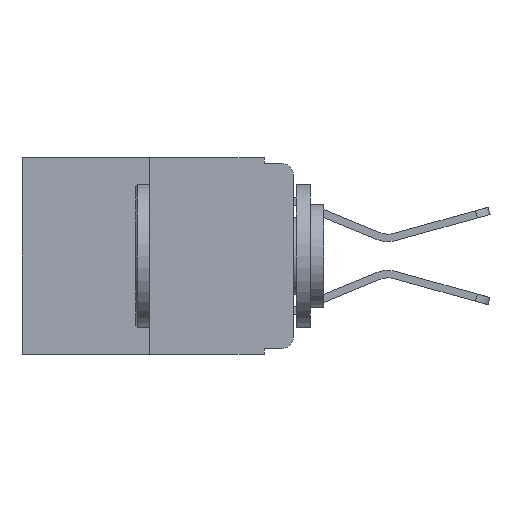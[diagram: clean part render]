
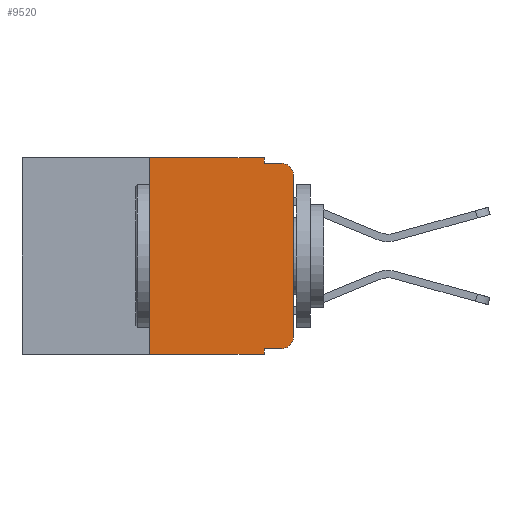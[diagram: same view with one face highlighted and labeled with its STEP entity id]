
A CAD part, left-side view. The second image highlights one B-rep face of the part: STEP entity #9520.
In plain terms, the highlighted planar face has unit normal (-1, 0, 0).
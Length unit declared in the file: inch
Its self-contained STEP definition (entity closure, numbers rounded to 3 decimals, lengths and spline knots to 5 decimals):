
#51 = DIRECTION ( 'NONE',  ( 0., 0., -1. ) ) ;
#485 = VECTOR ( 'NONE', #3410, 39.37008 ) ;
#599 = CARTESIAN_POINT ( 'NONE',  ( 0., 0.473, 0. ) ) ;
#651 = DIRECTION ( 'NONE',  ( 0., 0., 1. ) ) ;
#679 = VERTEX_POINT ( 'NONE', #16897 ) ;
#790 = EDGE_LOOP ( 'NONE', ( #5676, #9482, #6109, #9909, #6571, #10332, #13856, #10764, #17760, #11168 ) ) ;
#1125 = LINE ( 'NONE', #15892, #15273 ) ;
#1356 = CARTESIAN_POINT ( 'NONE',  ( 0., 0.051, -0.333 ) ) ;
#2352 = FACE_OUTER_BOUND ( 'NONE', #790, .T. ) ;
#2386 = VECTOR ( 'NONE', #51, 39.37008 ) ;
#2667 = CARTESIAN_POINT ( 'NONE',  ( 0., 0.25, 0. ) ) ;
#2975 = DIRECTION ( 'NONE',  ( 0., 0., -1. ) ) ;
#3064 = AXIS2_PLACEMENT_3D ( 'NONE', #599, #6646, #16149 ) ;
#3410 = DIRECTION ( 'NONE',  ( 0., -1., 0. ) ) ;
#3699 = CARTESIAN_POINT ( 'NONE',  ( 0., 0.25, -0.343 ) ) ;
#4577 = EDGE_CURVE ( 'NONE', #679, #4791, #16832, .T. ) ;
#4617 = CARTESIAN_POINT ( 'NONE',  ( 0., 0.051, -0.343 ) ) ;
#4672 = CARTESIAN_POINT ( 'NONE',  ( 0., 0., -0.03 ) ) ;
#4791 = VERTEX_POINT ( 'NONE', #8675 ) ;
#5560 = EDGE_CURVE ( 'NONE', #17378, #679, #10414, .T. ) ;
#5676 = ORIENTED_EDGE ( 'NONE', *, *, #11182, .T. ) ;
#6109 = ORIENTED_EDGE ( 'NONE', *, *, #9392, .F. ) ;
#6330 = VERTEX_POINT ( 'NONE', #2667 ) ;
#6506 = EDGE_CURVE ( 'NONE', #17378, #12170, #6618, .T. ) ;
#6571 = ORIENTED_EDGE ( 'NONE', *, *, #9517, .F. ) ;
#6618 = LINE ( 'NONE', #10194, #13485 ) ;
#6646 = DIRECTION ( 'NONE',  ( 1., 0., 0. ) ) ;
#6803 = CARTESIAN_POINT ( 'NONE',  ( 0., 0.02, -0.03 ) ) ;
#7354 = CARTESIAN_POINT ( 'NONE',  ( 0., 0., 0. ) ) ;
#7487 = EDGE_CURVE ( 'NONE', #8853, #6330, #9915, .T. ) ;
#7873 = CARTESIAN_POINT ( 'NONE',  ( 0., 0.473, -0.343 ) ) ;
#8002 = LINE ( 'NONE', #7873, #485 ) ;
#8190 = DIRECTION ( 'NONE',  ( -1., 0., 0. ) ) ;
#8303 = DIRECTION ( 'NONE',  ( 0., 0., -1. ) ) ;
#8476 = EDGE_CURVE ( 'NONE', #15116, #13767, #13199, .T. ) ;
#8675 = CARTESIAN_POINT ( 'NONE',  ( 0., 0., -0.313 ) ) ;
#8853 = VERTEX_POINT ( 'NONE', #3699 ) ;
#9007 = CARTESIAN_POINT ( 'NONE',  ( 0., 0.051, 0. ) ) ;
#9392 = EDGE_CURVE ( 'NONE', #13767, #12558, #1125, .T. ) ;
#9461 = CARTESIAN_POINT ( 'NONE',  ( 0., 0.473, 0. ) ) ;
#9482 = ORIENTED_EDGE ( 'NONE', *, *, #10296, .T. ) ;
#9517 = EDGE_CURVE ( 'NONE', #6330, #15116, #10914, .T. ) ;
#9520 = ADVANCED_FACE ( 'NONE', ( #2352 ), #14814, .F. ) ;
#9909 = ORIENTED_EDGE ( 'NONE', *, *, #8476, .F. ) ;
#9915 = LINE ( 'NONE', #16144, #15753 ) ;
#9991 = VECTOR ( 'NONE', #12642, 39.37008 ) ;
#10194 = CARTESIAN_POINT ( 'NONE',  ( 0., 0.051, 0. ) ) ;
#10296 = EDGE_CURVE ( 'NONE', #12800, #12558, #15470, .T. ) ;
#10332 = ORIENTED_EDGE ( 'NONE', *, *, #7487, .F. ) ;
#10414 = LINE ( 'NONE', #15318, #9991 ) ;
#10456 = VECTOR ( 'NONE', #11479, 39.37008 ) ;
#10764 = ORIENTED_EDGE ( 'NONE', *, *, #6506, .F. ) ;
#10914 = LINE ( 'NONE', #9461, #13587 ) ;
#11168 = ORIENTED_EDGE ( 'NONE', *, *, #4577, .T. ) ;
#11182 = EDGE_CURVE ( 'NONE', #4791, #12800, #14404, .T. ) ;
#11479 = DIRECTION ( 'NONE',  ( 0., 0., 1. ) ) ;
#11923 = AXIS2_PLACEMENT_3D ( 'NONE', #6803, #16303, #8303 ) ;
#12170 = VERTEX_POINT ( 'NONE', #4617 ) ;
#12172 = DIRECTION ( 'NONE',  ( 0., -1., 0. ) ) ;
#12365 = CARTESIAN_POINT ( 'NONE',  ( 0., 0.02, -0.01 ) ) ;
#12558 = VERTEX_POINT ( 'NONE', #12365 ) ;
#12642 = DIRECTION ( 'NONE',  ( 0., -1., 0. ) ) ;
#12800 = VERTEX_POINT ( 'NONE', #4672 ) ;
#13199 = LINE ( 'NONE', #9007, #2386 ) ;
#13485 = VECTOR ( 'NONE', #2975, 39.37008 ) ;
#13587 = VECTOR ( 'NONE', #12172, 39.37008 ) ;
#13752 = EDGE_CURVE ( 'NONE', #8853, #12170, #8002, .T. ) ;
#13767 = VERTEX_POINT ( 'NONE', #13834 ) ;
#13834 = CARTESIAN_POINT ( 'NONE',  ( 0., 0.051, -0.01 ) ) ;
#13856 = ORIENTED_EDGE ( 'NONE', *, *, #13752, .T. ) ;
#13916 = CARTESIAN_POINT ( 'NONE',  ( 0., 0.051, 0. ) ) ;
#14404 = LINE ( 'NONE', #7354, #10456 ) ;
#14814 = PLANE ( 'NONE',  #3064 ) ;
#15116 = VERTEX_POINT ( 'NONE', #13916 ) ;
#15188 = AXIS2_PLACEMENT_3D ( 'NONE', #16202, #8190, #17510 ) ;
#15273 = VECTOR ( 'NONE', #17172, 39.37008 ) ;
#15318 = CARTESIAN_POINT ( 'NONE',  ( 0., 0.051, -0.333 ) ) ;
#15470 = CIRCLE ( 'NONE', #11923, 0.02 ) ;
#15753 = VECTOR ( 'NONE', #651, 39.37008 ) ;
#15892 = CARTESIAN_POINT ( 'NONE',  ( 0., 0.051, -0.01 ) ) ;
#16144 = CARTESIAN_POINT ( 'NONE',  ( 0., 0.25, 0. ) ) ;
#16149 = DIRECTION ( 'NONE',  ( 0., 0., -1. ) ) ;
#16202 = CARTESIAN_POINT ( 'NONE',  ( 0., 0.02, -0.313 ) ) ;
#16303 = DIRECTION ( 'NONE',  ( -1., 0., 0. ) ) ;
#16832 = CIRCLE ( 'NONE', #15188, 0.02 ) ;
#16897 = CARTESIAN_POINT ( 'NONE',  ( 0., 0.02, -0.333 ) ) ;
#17172 = DIRECTION ( 'NONE',  ( 0., -1., 0. ) ) ;
#17378 = VERTEX_POINT ( 'NONE', #1356 ) ;
#17510 = DIRECTION ( 'NONE',  ( 0., 0., -1. ) ) ;
#17760 = ORIENTED_EDGE ( 'NONE', *, *, #5560, .T. ) ;
